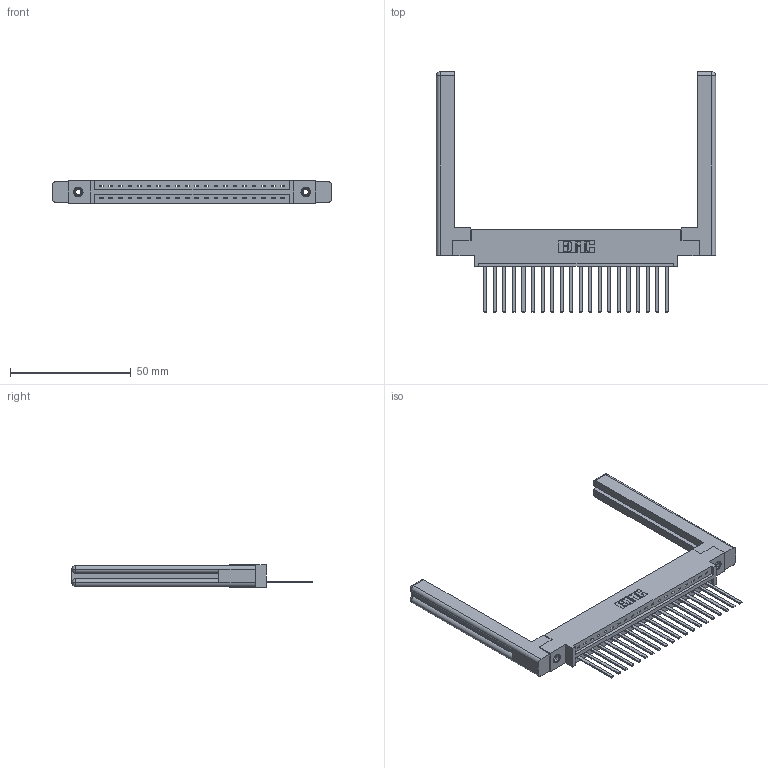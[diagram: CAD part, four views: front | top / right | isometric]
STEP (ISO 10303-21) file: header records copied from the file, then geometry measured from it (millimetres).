
FILE_DESCRIPTION (( 'STEP AP203' ), '1' );
FILE_NAME ('387-020-544-658.STEP', '2019-10-02T23:07:21', ( '' ), ( '' ), 'SwSTEP 2.0', 'SolidWorks 2016', '' );
FILE_SCHEMA (( 'CONFIG_CONTROL_DESIGN' ));
Length unit declared in the file: inch
Products named in the file (5): 345-250-001_345-250-001-102; 337 Part_0.170 Offset - 0.156 Dia-TI; 345-292-001_345-293-144; 387-020-544-658; 307-220-058
Assembly tree (25 placements, depth 2):
  387-020-544-658
    337 Part_0.170 Offset - 0.156 Dia-TI
    345-292-001_345-293-144  x20
    345-250-001_345-250-001-102  x2
    307-220-058  x2
Bounding box: 115.87 x 99.7 x 9.4 mm (x, y, z)
Volume: 19044.2 mm3; surface area: 18227.6 mm2
Topology: 25 solids, 25 shells, 1380 faces, 4077 edges, 2678 vertices
Faces by surface type: plane 998, cylinder 358, cone 12, torus 12
Entity records: 20294 total; most frequent: CARTESIAN_POINT 3533, ORIENTED_EDGE 3428, DIRECTION 3034, EDGE_CURVE 1714, VECTOR 1542, LINE 1542, VERTEX_POINT 1134, AXIS2_PLACEMENT_3D 746
